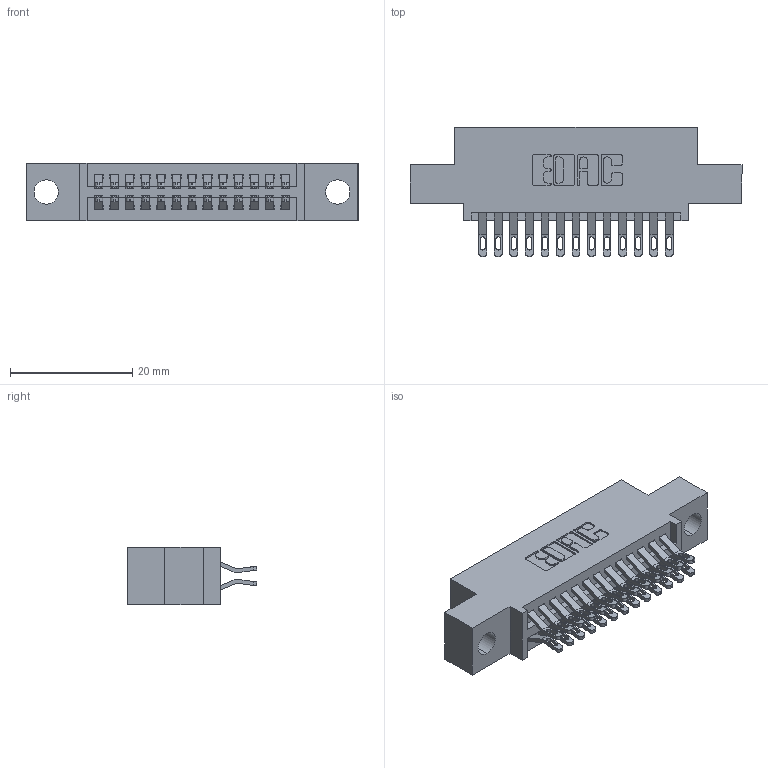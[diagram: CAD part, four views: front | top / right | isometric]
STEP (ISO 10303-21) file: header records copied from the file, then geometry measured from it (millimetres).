
FILE_DESCRIPTION (( 'STEP AP203' ), '1' );
FILE_NAME ('395-026-555-504.STEP', '2021-06-16T19:34:32', ( '' ), ( '' ), 'SwSTEP 2.0', 'SolidWorks 2020', '' );
FILE_SCHEMA (( 'CONFIG_CONTROL_DESIGN' ));
Length unit declared in the file: inch
Products named in the file (3): 345-292-001_555 Tail; 345 Part_0.110 Offset - 0.156 Dia-TI; 395-026-555-504
Assembly tree (27 placements, depth 2):
  395-026-555-504
    345 Part_0.110 Offset - 0.156 Dia-TI
    345-292-001_555 Tail  x26
Bounding box: 54.23 x 21.13 x 9.4 mm (x, y, z)
Volume: 4894.8 mm3; surface area: 6880.4 mm2
Topology: 27 solids, 27 shells, 1600 faces, 4991 edges, 3326 vertices
Faces by surface type: plane 904, cylinder 696
Entity records: 14981 total; most frequent: CARTESIAN_POINT 2580, ORIENTED_EDGE 2482, DIRECTION 2277, EDGE_CURVE 1241, VECTOR 1037, LINE 1037, VERTEX_POINT 826, AXIS2_PLACEMENT_3D 620
